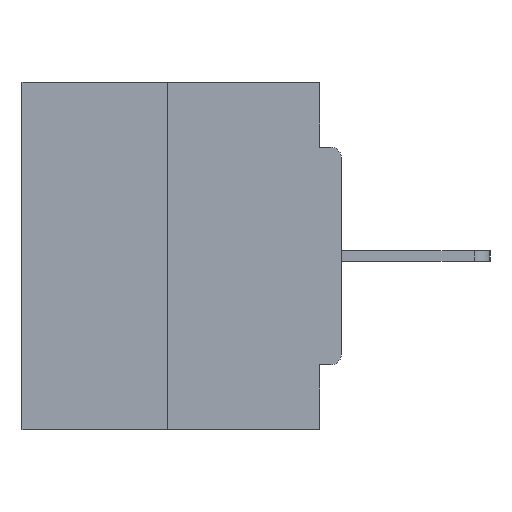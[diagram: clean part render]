
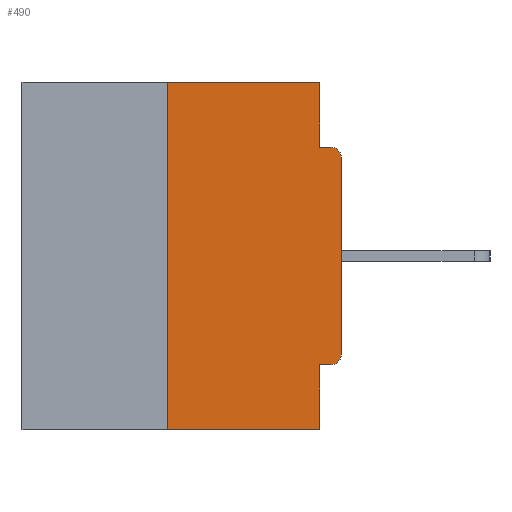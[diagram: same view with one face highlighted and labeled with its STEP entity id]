
A CAD part, left-side view. The second image highlights one B-rep face of the part: STEP entity #490.
In plain terms, the highlighted planar face has unit normal (-1, 0, 0).
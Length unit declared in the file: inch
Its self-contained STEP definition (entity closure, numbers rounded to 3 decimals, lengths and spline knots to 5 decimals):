
#490 = ADVANCED_FACE ( 'NONE', ( #4755 ), #15931, .F. ) ;
#1103 = CARTESIAN_POINT ( 'NONE',  ( 0., 0.25, 0. ) ) ;
#1616 = VERTEX_POINT ( 'NONE', #1103 ) ;
#1636 = VECTOR ( 'NONE', #11169, 39.37008 ) ;
#1676 = EDGE_LOOP ( 'NONE', ( #14473, #21336, #28758, #29577, #14467, #33727, #34387, #25913, #18934, #10087 ) ) ;
#2606 = CARTESIAN_POINT ( 'NONE',  ( 0., 0.015, -0.1085 ) ) ;
#3379 = CARTESIAN_POINT ( 'NONE',  ( 0., 0.015, -0.4065 ) ) ;
#3560 = VERTEX_POINT ( 'NONE', #17701 ) ;
#3652 = LINE ( 'NONE', #26623, #7236 ) ;
#4755 = FACE_OUTER_BOUND ( 'NONE', #1676, .T. ) ;
#4776 = DIRECTION ( 'NONE',  ( -1., 0., 0. ) ) ;
#5103 = AXIS2_PLACEMENT_3D ( 'NONE', #2606, #8797, #5861 ) ;
#5295 = CARTESIAN_POINT ( 'NONE',  ( 0., 0.031, -0.4065 ) ) ;
#5410 = DIRECTION ( 'NONE',  ( 0., 0., -1. ) ) ;
#5834 = CARTESIAN_POINT ( 'NONE',  ( 0., 0.015, -0.0935 ) ) ;
#5861 = DIRECTION ( 'NONE',  ( 0., 0., -1. ) ) ;
#5931 = EDGE_CURVE ( 'NONE', #6440, #25164, #25911, .T. ) ;
#6440 = VERTEX_POINT ( 'NONE', #3379 ) ;
#7072 = EDGE_CURVE ( 'NONE', #21392, #29684, #23148, .T. ) ;
#7236 = VECTOR ( 'NONE', #15209, 39.37008 ) ;
#7757 = VECTOR ( 'NONE', #28877, 39.37008 ) ;
#8022 = CIRCLE ( 'NONE', #5103, 0.015 ) ;
#8580 = EDGE_CURVE ( 'NONE', #3560, #26563, #3652, .T. ) ;
#8797 = DIRECTION ( 'NONE',  ( -1., 0., 0. ) ) ;
#9011 = VECTOR ( 'NONE', #5410, 39.37008 ) ;
#9232 = CARTESIAN_POINT ( 'NONE',  ( 0., 0.46, -0.5 ) ) ;
#9743 = CARTESIAN_POINT ( 'NONE',  ( 0., 0., -0.1085 ) ) ;
#9974 = AXIS2_PLACEMENT_3D ( 'NONE', #13517, #21791, #35942 ) ;
#10076 = AXIS2_PLACEMENT_3D ( 'NONE', #23882, #4776, #13002 ) ;
#10087 = ORIENTED_EDGE ( 'NONE', *, *, #15938, .F. ) ;
#11169 = DIRECTION ( 'NONE',  ( 0., 0., 1. ) ) ;
#12124 = DIRECTION ( 'NONE',  ( 0., 0., -1. ) ) ;
#12238 = CARTESIAN_POINT ( 'NONE',  ( 0., 0., -0.4065 ) ) ;
#12303 = EDGE_CURVE ( 'NONE', #6440, #21392, #19947, .T. ) ;
#13002 = DIRECTION ( 'NONE',  ( 0., 0., -1. ) ) ;
#13517 = CARTESIAN_POINT ( 'NONE',  ( 0., 0.46, 0. ) ) ;
#14467 = ORIENTED_EDGE ( 'NONE', *, *, #12303, .F. ) ;
#14470 = EDGE_CURVE ( 'NONE', #19712, #29684, #34398, .T. ) ;
#14473 = ORIENTED_EDGE ( 'NONE', *, *, #25707, .F. ) ;
#15209 = DIRECTION ( 'NONE',  ( 0., -1., 0. ) ) ;
#15931 = PLANE ( 'NONE',  #9974 ) ;
#15938 = EDGE_CURVE ( 'NONE', #24298, #3560, #21939, .T. ) ;
#16006 = EDGE_CURVE ( 'NONE', #19712, #1616, #30022, .T. ) ;
#16324 = CARTESIAN_POINT ( 'NONE',  ( 0., 0., 0. ) ) ;
#17701 = CARTESIAN_POINT ( 'NONE',  ( 0., 0.031, -0.0935 ) ) ;
#18583 = VECTOR ( 'NONE', #12124, 39.37008 ) ;
#18934 = ORIENTED_EDGE ( 'NONE', *, *, #8580, .F. ) ;
#19001 = CARTESIAN_POINT ( 'NONE',  ( 0., 0.25, 0. ) ) ;
#19044 = CARTESIAN_POINT ( 'NONE',  ( 0., 0., -0.3915 ) ) ;
#19533 = LINE ( 'NONE', #20268, #27745 ) ;
#19712 = VERTEX_POINT ( 'NONE', #36200 ) ;
#19947 = LINE ( 'NONE', #12238, #21606 ) ;
#20268 = CARTESIAN_POINT ( 'NONE',  ( 0., 0.46, 0. ) ) ;
#20310 = CARTESIAN_POINT ( 'NONE',  ( 0., 0.031, 0. ) ) ;
#20438 = CARTESIAN_POINT ( 'NONE',  ( 0., 0.031, -0.5 ) ) ;
#21336 = ORIENTED_EDGE ( 'NONE', *, *, #16006, .F. ) ;
#21392 = VERTEX_POINT ( 'NONE', #5295 ) ;
#21606 = VECTOR ( 'NONE', #22898, 39.37008 ) ;
#21791 = DIRECTION ( 'NONE',  ( 1., 0., 0. ) ) ;
#21939 = LINE ( 'NONE', #35895, #9011 ) ;
#22123 = DIRECTION ( 'NONE',  ( 0., 0., 1. ) ) ;
#22898 = DIRECTION ( 'NONE',  ( 0., 1., 0. ) ) ;
#23101 = VECTOR ( 'NONE', #22123, 39.37008 ) ;
#23148 = LINE ( 'NONE', #26462, #18583 ) ;
#23882 = CARTESIAN_POINT ( 'NONE',  ( 0., 0.015, -0.3915 ) ) ;
#24298 = VERTEX_POINT ( 'NONE', #20310 ) ;
#25164 = VERTEX_POINT ( 'NONE', #19044 ) ;
#25707 = EDGE_CURVE ( 'NONE', #1616, #24298, #19533, .T. ) ;
#25911 = CIRCLE ( 'NONE', #10076, 0.015 ) ;
#25913 = ORIENTED_EDGE ( 'NONE', *, *, #29277, .T. ) ;
#26462 = CARTESIAN_POINT ( 'NONE',  ( 0., 0.031, -0.5 ) ) ;
#26563 = VERTEX_POINT ( 'NONE', #5834 ) ;
#26623 = CARTESIAN_POINT ( 'NONE',  ( 0., 0., -0.0935 ) ) ;
#27745 = VECTOR ( 'NONE', #28188, 39.37008 ) ;
#27912 = LINE ( 'NONE', #16324, #1636 ) ;
#28188 = DIRECTION ( 'NONE',  ( 0., -1., 0. ) ) ;
#28758 = ORIENTED_EDGE ( 'NONE', *, *, #14470, .T. ) ;
#28877 = DIRECTION ( 'NONE',  ( 0., -1., 0. ) ) ;
#29277 = EDGE_CURVE ( 'NONE', #34564, #26563, #8022, .T. ) ;
#29577 = ORIENTED_EDGE ( 'NONE', *, *, #7072, .F. ) ;
#29684 = VERTEX_POINT ( 'NONE', #20438 ) ;
#30022 = LINE ( 'NONE', #19001, #23101 ) ;
#33727 = ORIENTED_EDGE ( 'NONE', *, *, #5931, .T. ) ;
#34387 = ORIENTED_EDGE ( 'NONE', *, *, #34628, .T. ) ;
#34398 = LINE ( 'NONE', #9232, #7757 ) ;
#34564 = VERTEX_POINT ( 'NONE', #9743 ) ;
#34628 = EDGE_CURVE ( 'NONE', #25164, #34564, #27912, .T. ) ;
#35895 = CARTESIAN_POINT ( 'NONE',  ( 0., 0.031, 0. ) ) ;
#35942 = DIRECTION ( 'NONE',  ( 0., 0., -1. ) ) ;
#36200 = CARTESIAN_POINT ( 'NONE',  ( 0., 0.25, -0.5 ) ) ;
